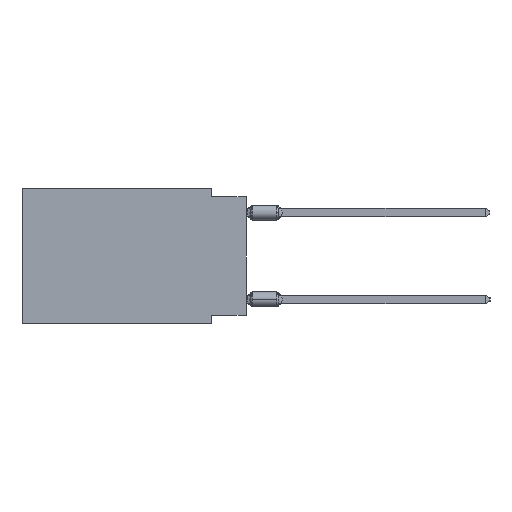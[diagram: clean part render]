
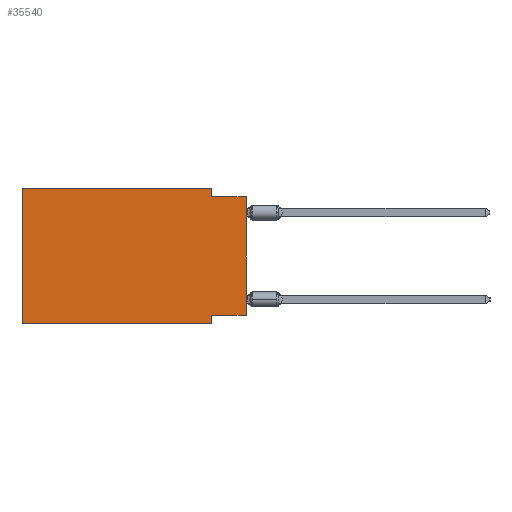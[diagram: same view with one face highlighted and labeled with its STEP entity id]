
A CAD part, left-side view. The second image highlights one B-rep face of the part: STEP entity #35540.
In plain terms, the highlighted planar face has unit normal (-1, 0, 0).
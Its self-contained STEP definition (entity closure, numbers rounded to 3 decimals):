
#335 = CARTESIAN_POINT ( 'NONE',  ( 0., 2.54, 0. ) ) ;
#778 = EDGE_CURVE ( 'NONE', #31927, #10659, #12302, .T. ) ;
#1166 = EDGE_CURVE ( 'NONE', #5780, #39608, #30218, .T. ) ;
#2693 = DIRECTION ( 'NONE',  ( 0., -1., 0. ) ) ;
#2924 = VERTEX_POINT ( 'NONE', #26356 ) ;
#3521 = VECTOR ( 'NONE', #21975, 1000. ) ;
#5780 = VERTEX_POINT ( 'NONE', #335 ) ;
#7357 = CARTESIAN_POINT ( 'NONE',  ( 0., 16.383, 0. ) ) ;
#7935 = CARTESIAN_POINT ( 'NONE',  ( 0., 16.383, 0. ) ) ;
#8471 = AXIS2_PLACEMENT_3D ( 'NONE', #42659, #34393, #23739 ) ;
#8590 = CARTESIAN_POINT ( 'NONE',  ( 0., 2.54, -0.635 ) ) ;
#10626 = VERTEX_POINT ( 'NONE', #11488 ) ;
#10659 = VERTEX_POINT ( 'NONE', #7357 ) ;
#11461 = ORIENTED_EDGE ( 'NONE', *, *, #29997, .T. ) ;
#11488 = CARTESIAN_POINT ( 'NONE',  ( 0., 0., -0.635 ) ) ;
#12302 = LINE ( 'NONE', #7935, #35576 ) ;
#12443 = VECTOR ( 'NONE', #19373, 1000. ) ;
#13953 = ORIENTED_EDGE ( 'NONE', *, *, #22154, .F. ) ;
#14113 = CARTESIAN_POINT ( 'NONE',  ( 0., 2.54, -9.271 ) ) ;
#14183 = CARTESIAN_POINT ( 'NONE',  ( 0., 2.54, -9.906 ) ) ;
#15968 = PLANE ( 'NONE',  #8471 ) ;
#16495 = VECTOR ( 'NONE', #27956, 1000. ) ;
#16563 = CARTESIAN_POINT ( 'NONE',  ( 0., 16.383, 0. ) ) ;
#17061 = EDGE_CURVE ( 'NONE', #31927, #2924, #41856, .T. ) ;
#18353 = CARTESIAN_POINT ( 'NONE',  ( 0., 0., -9.271 ) ) ;
#19282 = CARTESIAN_POINT ( 'NONE',  ( 0., 16.383, -9.906 ) ) ;
#19302 = DIRECTION ( 'NONE',  ( 0., 0., -1. ) ) ;
#19373 = DIRECTION ( 'NONE',  ( 0., 0., 1. ) ) ;
#19835 = VERTEX_POINT ( 'NONE', #18353 ) ;
#21680 = VERTEX_POINT ( 'NONE', #14113 ) ;
#21975 = DIRECTION ( 'NONE',  ( 0., 1., 0. ) ) ;
#22154 = EDGE_CURVE ( 'NONE', #39608, #10626, #31816, .T. ) ;
#22219 = CARTESIAN_POINT ( 'NONE',  ( 0., 0., -9.271 ) ) ;
#22753 = DIRECTION ( 'NONE',  ( 0., 0., 1. ) ) ;
#23379 = LINE ( 'NONE', #16563, #16495 ) ;
#23739 = DIRECTION ( 'NONE',  ( 0., 0., -1. ) ) ;
#24631 = CARTESIAN_POINT ( 'NONE',  ( 0., 16.383, -9.906 ) ) ;
#25357 = DIRECTION ( 'NONE',  ( 0., 0., -1. ) ) ;
#26356 = CARTESIAN_POINT ( 'NONE',  ( 0., 2.54, -9.906 ) ) ;
#26784 = EDGE_CURVE ( 'NONE', #19835, #21680, #28758, .T. ) ;
#27599 = FACE_OUTER_BOUND ( 'NONE', #44845, .T. ) ;
#27645 = ORIENTED_EDGE ( 'NONE', *, *, #33288, .F. ) ;
#27956 = DIRECTION ( 'NONE',  ( 0., -1., 0. ) ) ;
#28180 = CARTESIAN_POINT ( 'NONE',  ( 0., 0., -0.635 ) ) ;
#28758 = LINE ( 'NONE', #22219, #3521 ) ;
#29180 = VECTOR ( 'NONE', #37461, 1000. ) ;
#29997 = EDGE_CURVE ( 'NONE', #19835, #10626, #41462, .T. ) ;
#30218 = LINE ( 'NONE', #33598, #38678 ) ;
#30750 = ORIENTED_EDGE ( 'NONE', *, *, #17061, .T. ) ;
#31666 = ORIENTED_EDGE ( 'NONE', *, *, #778, .F. ) ;
#31816 = LINE ( 'NONE', #28180, #40455 ) ;
#31927 = VERTEX_POINT ( 'NONE', #24631 ) ;
#32182 = EDGE_CURVE ( 'NONE', #10659, #5780, #23379, .T. ) ;
#33288 = EDGE_CURVE ( 'NONE', #21680, #2924, #36255, .T. ) ;
#33598 = CARTESIAN_POINT ( 'NONE',  ( 0., 2.54, 0. ) ) ;
#34393 = DIRECTION ( 'NONE',  ( 1., 0., 0. ) ) ;
#35540 = ADVANCED_FACE ( 'NONE', ( #27599 ), #15968, .F. ) ;
#35576 = VECTOR ( 'NONE', #22753, 1000. ) ;
#36255 = LINE ( 'NONE', #14183, #42182 ) ;
#37461 = DIRECTION ( 'NONE',  ( 0., -1., 0. ) ) ;
#37804 = CARTESIAN_POINT ( 'NONE',  ( 0., 0., 0. ) ) ;
#38678 = VECTOR ( 'NONE', #19302, 1000. ) ;
#39608 = VERTEX_POINT ( 'NONE', #8590 ) ;
#40455 = VECTOR ( 'NONE', #2693, 1000. ) ;
#41462 = LINE ( 'NONE', #37804, #12443 ) ;
#41856 = LINE ( 'NONE', #19282, #29180 ) ;
#42182 = VECTOR ( 'NONE', #25357, 1000. ) ;
#42659 = CARTESIAN_POINT ( 'NONE',  ( 0., 16.383, 0. ) ) ;
#44845 = EDGE_LOOP ( 'NONE', ( #11461, #13953, #46341, #46322, #31666, #30750, #27645, #47165 ) ) ;
#46322 = ORIENTED_EDGE ( 'NONE', *, *, #32182, .F. ) ;
#46341 = ORIENTED_EDGE ( 'NONE', *, *, #1166, .F. ) ;
#47165 = ORIENTED_EDGE ( 'NONE', *, *, #26784, .F. ) ;
